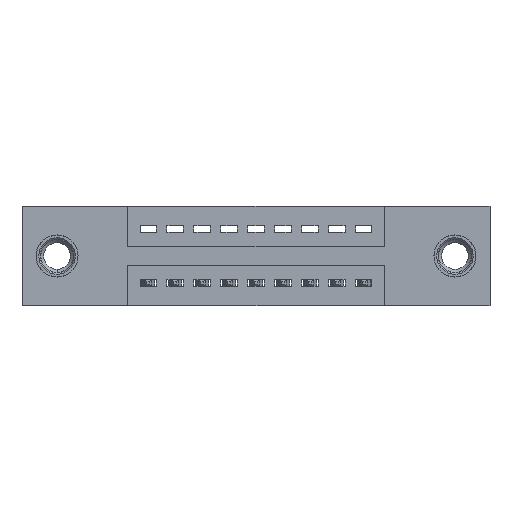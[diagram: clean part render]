
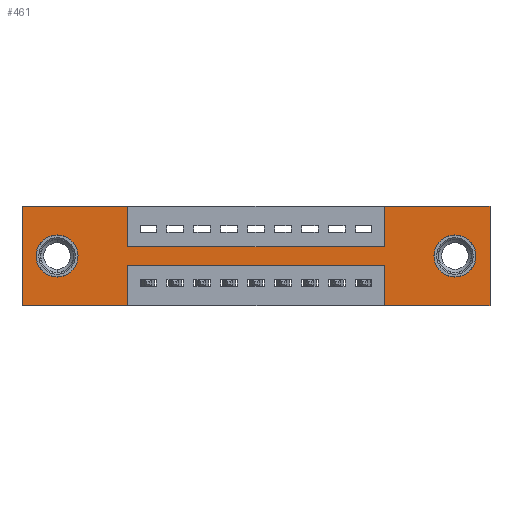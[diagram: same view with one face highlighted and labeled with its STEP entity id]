
A CAD part, front view. The second image highlights one B-rep face of the part: STEP entity #461.
In plain terms, the highlighted planar face has unit normal (0, -1, 0).
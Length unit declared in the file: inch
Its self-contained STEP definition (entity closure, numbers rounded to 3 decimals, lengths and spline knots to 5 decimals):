
#5 = CARTESIAN_POINT ( 'NONE',  ( 1.3425, 0., 0. ) ) ;
#86 = DIRECTION ( 'NONE',  ( 0., 0., 1. ) ) ;
#166 = VERTEX_POINT ( 'NONE', #1980 ) ;
#243 = VECTOR ( 'NONE', #10020, 39.37008 ) ;
#270 = CARTESIAN_POINT ( 'NONE',  ( 0.13, 0., -0.263 ) ) ;
#289 = LINE ( 'NONE', #7140, #10073 ) ;
#397 = DIRECTION ( 'NONE',  ( 0., 1., 0. ) ) ;
#422 = LINE ( 'NONE', #9551, #7926 ) ;
#461 = ADVANCED_FACE ( 'NONE', ( #10187, #10328, #2020 ), #1347, .T. ) ;
#468 = CARTESIAN_POINT ( 'NONE',  ( 1.3425, 0., -0.37 ) ) ;
#683 = AXIS2_PLACEMENT_3D ( 'NONE', #10444, #8527, #4704 ) ;
#686 = EDGE_CURVE ( 'NONE', #7923, #11243, #11484, .T. ) ;
#766 = LINE ( 'NONE', #2546, #10261 ) ;
#773 = EDGE_LOOP ( 'NONE', ( #1685, #11755, #11835, #2723, #11782, #8019, #7452, #4720, #11972, #4044, #2749, #9385 ) ) ;
#911 = AXIS2_PLACEMENT_3D ( 'NONE', #9153, #3403, #8110 ) ;
#1141 = CARTESIAN_POINT ( 'NONE',  ( 0.3925, 0., 0. ) ) ;
#1253 = LINE ( 'NONE', #11885, #4742 ) ;
#1310 = VERTEX_POINT ( 'NONE', #11144 ) ;
#1344 = DIRECTION ( 'NONE',  ( 0., 0., 1. ) ) ;
#1347 = PLANE ( 'NONE',  #8432 ) ;
#1438 = DIRECTION ( 'NONE',  ( 0., 0., -1. ) ) ;
#1685 = ORIENTED_EDGE ( 'NONE', *, *, #1952, .F. ) ;
#1700 = EDGE_CURVE ( 'NONE', #2057, #7923, #8024, .T. ) ;
#1722 = EDGE_CURVE ( 'NONE', #10267, #1310, #6103, .T. ) ;
#1817 = VERTEX_POINT ( 'NONE', #10603 ) ;
#1952 = EDGE_CURVE ( 'NONE', #3484, #10267, #1253, .T. ) ;
#1980 = CARTESIAN_POINT ( 'NONE',  ( 1.3425, 0., -0.22 ) ) ;
#2005 = VERTEX_POINT ( 'NONE', #468 ) ;
#2009 = EDGE_CURVE ( 'NONE', #11243, #2540, #8769, .T. ) ;
#2020 = FACE_OUTER_BOUND ( 'NONE', #773, .T. ) ;
#2057 = VERTEX_POINT ( 'NONE', #3369 ) ;
#2163 = VERTEX_POINT ( 'NONE', #11044 ) ;
#2210 = CARTESIAN_POINT ( 'NONE',  ( 0., 0., -0.37 ) ) ;
#2255 = ORIENTED_EDGE ( 'NONE', *, *, #7753, .T. ) ;
#2266 = AXIS2_PLACEMENT_3D ( 'NONE', #11339, #4508, #6575 ) ;
#2540 = VERTEX_POINT ( 'NONE', #4694 ) ;
#2546 = CARTESIAN_POINT ( 'NONE',  ( 0., 0., 0. ) ) ;
#2723 = ORIENTED_EDGE ( 'NONE', *, *, #6013, .F. ) ;
#2727 = CARTESIAN_POINT ( 'NONE',  ( 0.3925, 0., 0. ) ) ;
#2749 = ORIENTED_EDGE ( 'NONE', *, *, #12142, .F. ) ;
#3019 = AXIS2_PLACEMENT_3D ( 'NONE', #9990, #397, #11822 ) ;
#3230 = CARTESIAN_POINT ( 'NONE',  ( 0., 0., 0. ) ) ;
#3369 = CARTESIAN_POINT ( 'NONE',  ( 1.3425, 0., -0.15 ) ) ;
#3403 = DIRECTION ( 'NONE',  ( 0., 1., 0. ) ) ;
#3484 = VERTEX_POINT ( 'NONE', #10719 ) ;
#3707 = DIRECTION ( 'NONE',  ( 0., 0., -1. ) ) ;
#3937 = CARTESIAN_POINT ( 'NONE',  ( 1.3425, 0., 0. ) ) ;
#3971 = CARTESIAN_POINT ( 'NONE',  ( 0.13, 0., -0.107 ) ) ;
#4018 = CARTESIAN_POINT ( 'NONE',  ( 1.605, 0., -0.263 ) ) ;
#4044 = ORIENTED_EDGE ( 'NONE', *, *, #10525, .F. ) ;
#4154 = CARTESIAN_POINT ( 'NONE',  ( 1.735, 0., 0. ) ) ;
#4209 = ORIENTED_EDGE ( 'NONE', *, *, #11102, .T. ) ;
#4233 = LINE ( 'NONE', #3230, #12027 ) ;
#4385 = EDGE_CURVE ( 'NONE', #7121, #6139, #10840, .T. ) ;
#4392 = EDGE_CURVE ( 'NONE', #9139, #2163, #4705, .T. ) ;
#4508 = DIRECTION ( 'NONE',  ( 0., 1., 0. ) ) ;
#4694 = CARTESIAN_POINT ( 'NONE',  ( 1.735, 0., -0.37 ) ) ;
#4704 = DIRECTION ( 'NONE',  ( 0., 0., -1. ) ) ;
#4705 = LINE ( 'NONE', #2727, #5762 ) ;
#4720 = ORIENTED_EDGE ( 'NONE', *, *, #6635, .F. ) ;
#4742 = VECTOR ( 'NONE', #11928, 39.37008 ) ;
#5074 = DIRECTION ( 'NONE',  ( -1., 0., 0. ) ) ;
#5268 = CARTESIAN_POINT ( 'NONE',  ( 0., 0., -0.37 ) ) ;
#5664 = EDGE_LOOP ( 'NONE', ( #8181, #2255 ) ) ;
#5762 = VECTOR ( 'NONE', #3707, 39.37008 ) ;
#5777 = EDGE_LOOP ( 'NONE', ( #6905, #4209 ) ) ;
#6013 = EDGE_CURVE ( 'NONE', #2540, #2005, #12169, .T. ) ;
#6052 = LINE ( 'NONE', #7729, #9475 ) ;
#6103 = LINE ( 'NONE', #2210, #11929 ) ;
#6139 = VERTEX_POINT ( 'NONE', #4018 ) ;
#6575 = DIRECTION ( 'NONE',  ( 0., 0., -1. ) ) ;
#6635 = EDGE_CURVE ( 'NONE', #2163, #2057, #422, .T. ) ;
#6905 = ORIENTED_EDGE ( 'NONE', *, *, #7368, .T. ) ;
#7014 = CIRCLE ( 'NONE', #2266, 0.078 ) ;
#7121 = VERTEX_POINT ( 'NONE', #9720 ) ;
#7140 = CARTESIAN_POINT ( 'NONE',  ( 1.3425, 0., -0.37 ) ) ;
#7237 = CARTESIAN_POINT ( 'NONE',  ( 1.735, 0., 0. ) ) ;
#7368 = EDGE_CURVE ( 'NONE', #10411, #12063, #12256, .T. ) ;
#7452 = ORIENTED_EDGE ( 'NONE', *, *, #1700, .F. ) ;
#7729 = CARTESIAN_POINT ( 'NONE',  ( 0.3925, 0., -0.22 ) ) ;
#7753 = EDGE_CURVE ( 'NONE', #6139, #7121, #7014, .T. ) ;
#7923 = VERTEX_POINT ( 'NONE', #3937 ) ;
#7926 = VECTOR ( 'NONE', #10575, 39.37008 ) ;
#7949 = VECTOR ( 'NONE', #8549, 39.37008 ) ;
#7969 = DIRECTION ( 'NONE',  ( -1., 0., 0. ) ) ;
#8019 = ORIENTED_EDGE ( 'NONE', *, *, #686, .F. ) ;
#8024 = LINE ( 'NONE', #5, #11311 ) ;
#8110 = DIRECTION ( 'NONE',  ( 0., 0., 1. ) ) ;
#8181 = ORIENTED_EDGE ( 'NONE', *, *, #4385, .T. ) ;
#8432 = AXIS2_PLACEMENT_3D ( 'NONE', #5268, #9093, #1438 ) ;
#8527 = DIRECTION ( 'NONE',  ( 0., 1., 0. ) ) ;
#8549 = DIRECTION ( 'NONE',  ( -1., 0., 0. ) ) ;
#8623 = CARTESIAN_POINT ( 'NONE',  ( 0.3925, 0., -0.37 ) ) ;
#8769 = LINE ( 'NONE', #7237, #10448 ) ;
#9093 = DIRECTION ( 'NONE',  ( 0., -1., 0. ) ) ;
#9139 = VERTEX_POINT ( 'NONE', #1141 ) ;
#9153 = CARTESIAN_POINT ( 'NONE',  ( 0.13, 0., -0.185 ) ) ;
#9192 = DIRECTION ( 'NONE',  ( 0., 0., -1. ) ) ;
#9226 = DIRECTION ( 'NONE',  ( 1., 0., 0. ) ) ;
#9385 = ORIENTED_EDGE ( 'NONE', *, *, #1722, .F. ) ;
#9475 = VECTOR ( 'NONE', #7969, 39.37008 ) ;
#9551 = CARTESIAN_POINT ( 'NONE',  ( 0.3925, 0., -0.15 ) ) ;
#9720 = CARTESIAN_POINT ( 'NONE',  ( 1.605, 0., -0.107 ) ) ;
#9990 = CARTESIAN_POINT ( 'NONE',  ( 0.13, 0., -0.185 ) ) ;
#10020 = DIRECTION ( 'NONE',  ( 1., 0., 0. ) ) ;
#10073 = VECTOR ( 'NONE', #1344, 39.37008 ) ;
#10187 = FACE_BOUND ( 'NONE', #5664, .T. ) ;
#10261 = VECTOR ( 'NONE', #9226, 39.37008 ) ;
#10267 = VERTEX_POINT ( 'NONE', #8623 ) ;
#10328 = FACE_BOUND ( 'NONE', #5777, .T. ) ;
#10411 = VERTEX_POINT ( 'NONE', #3971 ) ;
#10444 = CARTESIAN_POINT ( 'NONE',  ( 1.605, 0., -0.185 ) ) ;
#10448 = VECTOR ( 'NONE', #9192, 39.37008 ) ;
#10525 = EDGE_CURVE ( 'NONE', #1817, #9139, #766, .T. ) ;
#10542 = CIRCLE ( 'NONE', #3019, 0.078 ) ;
#10575 = DIRECTION ( 'NONE',  ( 1., 0., 0. ) ) ;
#10603 = CARTESIAN_POINT ( 'NONE',  ( 0., 0., 0. ) ) ;
#10719 = CARTESIAN_POINT ( 'NONE',  ( 0.3925, 0., -0.22 ) ) ;
#10840 = CIRCLE ( 'NONE', #683, 0.078 ) ;
#10985 = EDGE_CURVE ( 'NONE', #166, #3484, #6052, .T. ) ;
#11044 = CARTESIAN_POINT ( 'NONE',  ( 0.3925, 0., -0.15 ) ) ;
#11102 = EDGE_CURVE ( 'NONE', #12063, #10411, #10542, .T. ) ;
#11144 = CARTESIAN_POINT ( 'NONE',  ( 0., 0., -0.37 ) ) ;
#11243 = VERTEX_POINT ( 'NONE', #4154 ) ;
#11311 = VECTOR ( 'NONE', #86, 39.37008 ) ;
#11339 = CARTESIAN_POINT ( 'NONE',  ( 1.605, 0., -0.185 ) ) ;
#11484 = LINE ( 'NONE', #11807, #243 ) ;
#11755 = ORIENTED_EDGE ( 'NONE', *, *, #10985, .F. ) ;
#11782 = ORIENTED_EDGE ( 'NONE', *, *, #2009, .F. ) ;
#11807 = CARTESIAN_POINT ( 'NONE',  ( 0., 0., 0. ) ) ;
#11822 = DIRECTION ( 'NONE',  ( 0., 0., 1. ) ) ;
#11835 = ORIENTED_EDGE ( 'NONE', *, *, #12312, .F. ) ;
#11885 = CARTESIAN_POINT ( 'NONE',  ( 0.3925, 0., -0.37 ) ) ;
#11928 = DIRECTION ( 'NONE',  ( 0., 0., -1. ) ) ;
#11929 = VECTOR ( 'NONE', #5074, 39.37008 ) ;
#11931 = CARTESIAN_POINT ( 'NONE',  ( 0., 0., -0.37 ) ) ;
#11969 = DIRECTION ( 'NONE',  ( 0., 0., 1. ) ) ;
#11972 = ORIENTED_EDGE ( 'NONE', *, *, #4392, .F. ) ;
#12027 = VECTOR ( 'NONE', #11969, 39.37008 ) ;
#12063 = VERTEX_POINT ( 'NONE', #270 ) ;
#12142 = EDGE_CURVE ( 'NONE', #1310, #1817, #4233, .T. ) ;
#12169 = LINE ( 'NONE', #11931, #7949 ) ;
#12256 = CIRCLE ( 'NONE', #911, 0.078 ) ;
#12312 = EDGE_CURVE ( 'NONE', #2005, #166, #289, .T. ) ;
